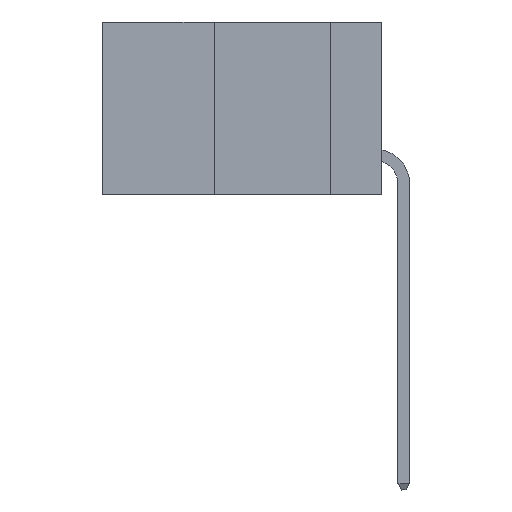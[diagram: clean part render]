
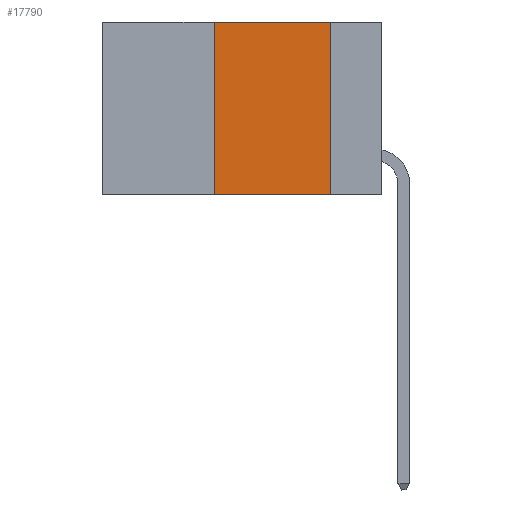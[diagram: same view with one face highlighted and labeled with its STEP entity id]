
A CAD part, left-side view. The second image highlights one B-rep face of the part: STEP entity #17790.
In plain terms, the highlighted planar face has unit normal (-1, 0, 0).
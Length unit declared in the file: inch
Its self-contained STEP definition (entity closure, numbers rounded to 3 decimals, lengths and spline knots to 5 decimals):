
#319 = VECTOR ( 'NONE', #36518, 39.37008 ) ;
#835 = CARTESIAN_POINT ( 'NONE',  ( 0., 0.6, -0.37 ) ) ;
#910 = FACE_OUTER_BOUND ( 'NONE', #23913, .T. ) ;
#1526 = CARTESIAN_POINT ( 'NONE',  ( 0., 0.11, 0. ) ) ;
#1871 = DIRECTION ( 'NONE',  ( 0., 0., -1. ) ) ;
#2307 = VERTEX_POINT ( 'NONE', #1526 ) ;
#3723 = DIRECTION ( 'NONE',  ( 0., -1., 0. ) ) ;
#3996 = LINE ( 'NONE', #4252, #32906 ) ;
#4252 = CARTESIAN_POINT ( 'NONE',  ( 0., 0.11, 0. ) ) ;
#4352 = DIRECTION ( 'NONE',  ( 0., 0., 1. ) ) ;
#6681 = LINE ( 'NONE', #33236, #20954 ) ;
#7593 = VERTEX_POINT ( 'NONE', #34279 ) ;
#8503 = CARTESIAN_POINT ( 'NONE',  ( 0., 0.11, -0.37 ) ) ;
#8585 = ORIENTED_EDGE ( 'NONE', *, *, #33668, .F. ) ;
#9751 = ORIENTED_EDGE ( 'NONE', *, *, #33316, .F. ) ;
#10221 = CARTESIAN_POINT ( 'NONE',  ( 0., 0.36, 0. ) ) ;
#11461 = ORIENTED_EDGE ( 'NONE', *, *, #33125, .T. ) ;
#12023 = LINE ( 'NONE', #10221, #32638 ) ;
#12740 = DIRECTION ( 'NONE',  ( 0., 0., -1. ) ) ;
#15048 = AXIS2_PLACEMENT_3D ( 'NONE', #36627, #15691, #12740 ) ;
#15691 = DIRECTION ( 'NONE',  ( 1., 0., 0. ) ) ;
#17790 = ADVANCED_FACE ( 'NONE', ( #910 ), #33662, .F. ) ;
#20620 = ORIENTED_EDGE ( 'NONE', *, *, #31237, .F. ) ;
#20954 = VECTOR ( 'NONE', #3723, 39.37008 ) ;
#23913 = EDGE_LOOP ( 'NONE', ( #8585, #9751, #20620, #11461 ) ) ;
#24162 = LINE ( 'NONE', #835, #319 ) ;
#31237 = EDGE_CURVE ( 'NONE', #34068, #7593, #12023, .T. ) ;
#32638 = VECTOR ( 'NONE', #4352, 39.37008 ) ;
#32906 = VECTOR ( 'NONE', #1871, 39.37008 ) ;
#33125 = EDGE_CURVE ( 'NONE', #34068, #34884, #24162, .T. ) ;
#33236 = CARTESIAN_POINT ( 'NONE',  ( 0., 0.6, 0. ) ) ;
#33316 = EDGE_CURVE ( 'NONE', #7593, #2307, #6681, .T. ) ;
#33662 = PLANE ( 'NONE',  #15048 ) ;
#33668 = EDGE_CURVE ( 'NONE', #2307, #34884, #3996, .T. ) ;
#34068 = VERTEX_POINT ( 'NONE', #34999 ) ;
#34279 = CARTESIAN_POINT ( 'NONE',  ( 0., 0.36, 0. ) ) ;
#34884 = VERTEX_POINT ( 'NONE', #8503 ) ;
#34999 = CARTESIAN_POINT ( 'NONE',  ( 0., 0.36, -0.37 ) ) ;
#36518 = DIRECTION ( 'NONE',  ( 0., -1., 0. ) ) ;
#36627 = CARTESIAN_POINT ( 'NONE',  ( 0., 0.6, 0. ) ) ;
